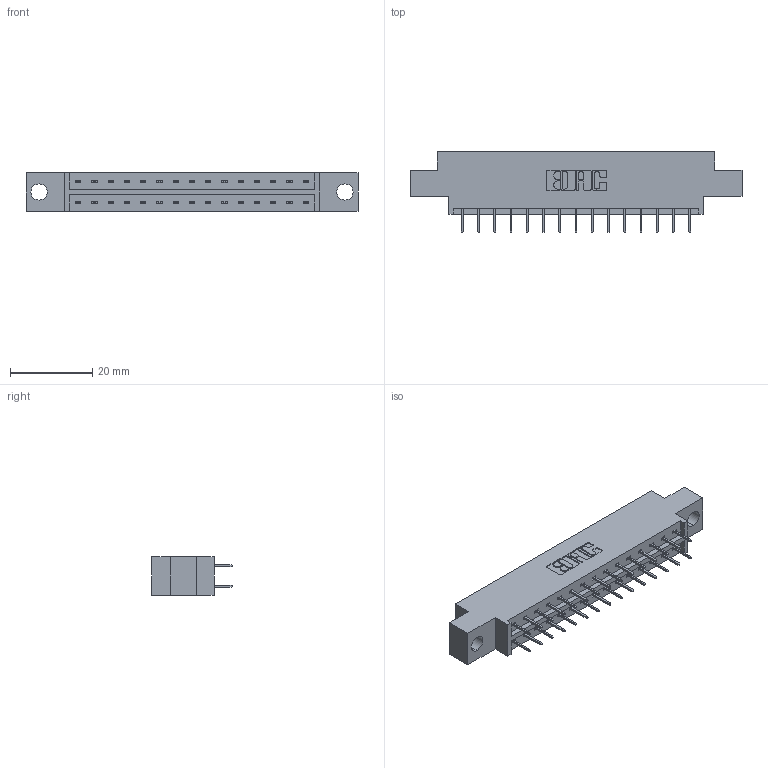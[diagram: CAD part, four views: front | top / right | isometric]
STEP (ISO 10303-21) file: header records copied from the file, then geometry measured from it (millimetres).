
FILE_DESCRIPTION (( 'STEP AP203' ), '1' );
FILE_NAME ('833-030-524-804.STEP', '2020-06-02T12:51:21', ( '' ), ( '' ), 'SwSTEP 2.0', 'SolidWorks 2020', '' );
FILE_SCHEMA (( 'CONFIG_CONTROL_DESIGN' ));
Length unit declared in the file: inch
Products named in the file (3): 833 Part_Offset - .156 Dia - TH; 833-030-524-804; 345-292-001_345-293-124
Assembly tree (31 placements, depth 2):
  833-030-524-804
    833 Part_Offset - .156 Dia - TH
    345-292-001_345-293-124  x30
Bounding box: 80.98 x 19.69 x 9.4 mm (x, y, z)
Volume: 7653.6 mm3; surface area: 8642.3 mm2
Topology: 31 solids, 31 shells, 1798 faces, 5093 edges, 3274 vertices
Faces by surface type: plane 1334, cylinder 464
Entity records: 13351 total; most frequent: CARTESIAN_POINT 2246, ORIENTED_EDGE 2182, DIRECTION 1967, EDGE_CURVE 1091, VECTOR 967, LINE 967, VERTEX_POINT 722, AXIS2_PLACEMENT_3D 500
